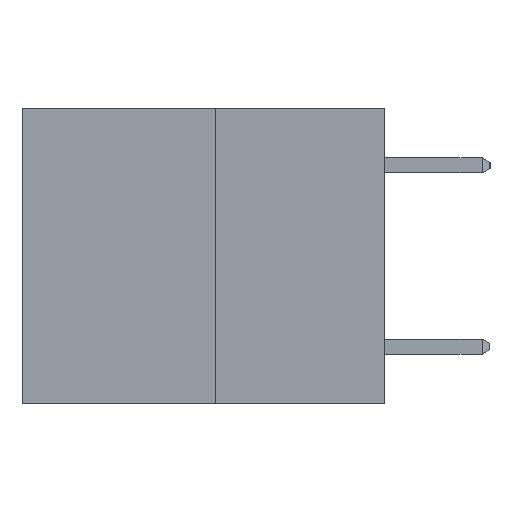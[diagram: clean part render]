
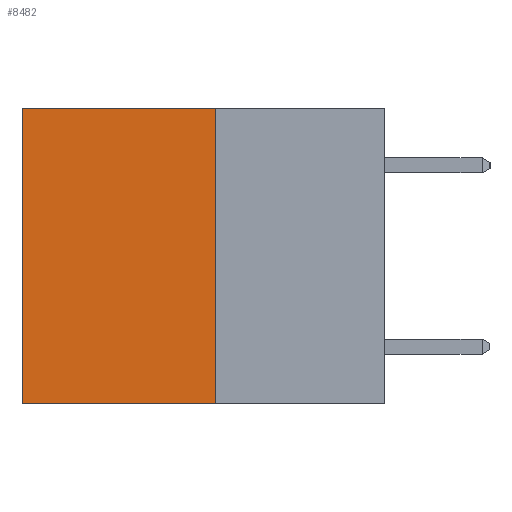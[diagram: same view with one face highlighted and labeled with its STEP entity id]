
A CAD part, left-side view. The second image highlights one B-rep face of the part: STEP entity #8482.
In plain terms, the highlighted planar face has unit normal (-1, 0, 0).
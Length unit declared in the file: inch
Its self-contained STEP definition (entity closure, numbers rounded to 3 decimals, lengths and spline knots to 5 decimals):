
#126 = LINE ( 'NONE', #8863, #9831 ) ;
#804 = DIRECTION ( 'NONE',  ( 0., 0., -1. ) ) ;
#1236 = VERTEX_POINT ( 'NONE', #5959 ) ;
#1269 = DIRECTION ( 'NONE',  ( 0., 0., -1. ) ) ;
#1537 = CARTESIAN_POINT ( 'NONE',  ( 0.3165, 0.28, -0.49 ) ) ;
#1891 = AXIS2_PLACEMENT_3D ( 'NONE', #2324, #3362, #11693 ) ;
#2324 = CARTESIAN_POINT ( 'NONE',  ( 0.3165, 0.28, -0.49 ) ) ;
#2848 = CARTESIAN_POINT ( 'NONE',  ( 0.3165, 0.6, -0.49 ) ) ;
#3215 = ORIENTED_EDGE ( 'NONE', *, *, #4971, .F. ) ;
#3242 = DIRECTION ( 'NONE',  ( 0., 1., 0. ) ) ;
#3362 = DIRECTION ( 'NONE',  ( 1., 0., 0. ) ) ;
#3792 = VERTEX_POINT ( 'NONE', #1537 ) ;
#4365 = LINE ( 'NONE', #7908, #4961 ) ;
#4775 = CARTESIAN_POINT ( 'NONE',  ( 0.3165, 0.28, 0. ) ) ;
#4961 = VECTOR ( 'NONE', #1269, 39.37008 ) ;
#4971 = EDGE_CURVE ( 'NONE', #5100, #3792, #5451, .T. ) ;
#5100 = VERTEX_POINT ( 'NONE', #4775 ) ;
#5451 = LINE ( 'NONE', #11713, #9733 ) ;
#5959 = CARTESIAN_POINT ( 'NONE',  ( 0.3165, 0.6, 0. ) ) ;
#6116 = EDGE_LOOP ( 'NONE', ( #10228, #10452, #3215, #7204 ) ) ;
#6747 = EDGE_CURVE ( 'NONE', #3792, #10424, #126, .T. ) ;
#7204 = ORIENTED_EDGE ( 'NONE', *, *, #9838, .T. ) ;
#7786 = DIRECTION ( 'NONE',  ( 0., 1., 0. ) ) ;
#7908 = CARTESIAN_POINT ( 'NONE',  ( 0.3165, 0.6, -0.49 ) ) ;
#7911 = CARTESIAN_POINT ( 'NONE',  ( 0.3165, 0.28, 0. ) ) ;
#8259 = EDGE_CURVE ( 'NONE', #1236, #10424, #4365, .T. ) ;
#8482 = ADVANCED_FACE ( 'NONE', ( #11979 ), #10811, .F. ) ;
#8863 = CARTESIAN_POINT ( 'NONE',  ( 0.3165, 0.28, -0.49 ) ) ;
#8871 = VECTOR ( 'NONE', #7786, 39.37008 ) ;
#9733 = VECTOR ( 'NONE', #804, 39.37008 ) ;
#9831 = VECTOR ( 'NONE', #3242, 39.37008 ) ;
#9838 = EDGE_CURVE ( 'NONE', #5100, #1236, #10655, .T. ) ;
#10228 = ORIENTED_EDGE ( 'NONE', *, *, #8259, .T. ) ;
#10424 = VERTEX_POINT ( 'NONE', #2848 ) ;
#10452 = ORIENTED_EDGE ( 'NONE', *, *, #6747, .F. ) ;
#10655 = LINE ( 'NONE', #7911, #8871 ) ;
#10811 = PLANE ( 'NONE',  #1891 ) ;
#11693 = DIRECTION ( 'NONE',  ( 0., 0., -1. ) ) ;
#11713 = CARTESIAN_POINT ( 'NONE',  ( 0.3165, 0.28, -0.49 ) ) ;
#11979 = FACE_OUTER_BOUND ( 'NONE', #6116, .T. ) ;
